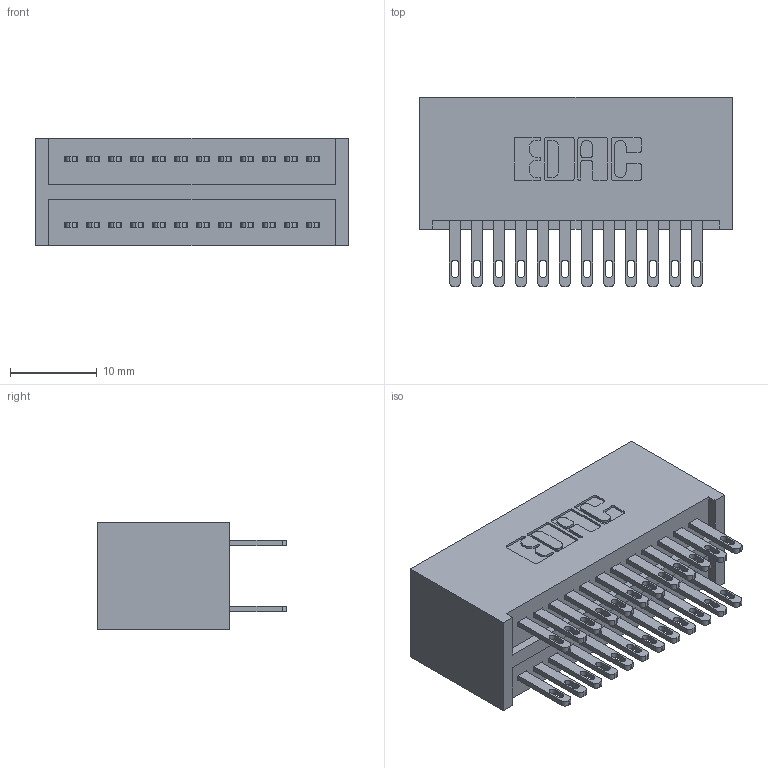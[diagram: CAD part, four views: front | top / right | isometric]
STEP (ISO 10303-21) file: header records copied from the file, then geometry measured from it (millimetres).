
FILE_DESCRIPTION (( 'STEP AP203' ), '1' );
FILE_NAME ('325-024-500-201.STEP', '2020-02-24T17:46:23', ( '' ), ( '' ), 'SwSTEP 2.0', 'SolidWorks 2016', '' );
FILE_SCHEMA (( 'CONFIG_CONTROL_DESIGN' ));
Length unit declared in the file: inch
Products named in the file (3): 325 Part_Lugless; 325-024-500-201; 325-292-001_325-293-100
Assembly tree (25 placements, depth 2):
  325-024-500-201
    325 Part_Lugless
    325-292-001_325-293-100  x24
Bounding box: 36.12 x 21.84 x 12.45 mm (x, y, z)
Volume: 5073.1 mm3; surface area: 6340.9 mm2
Topology: 25 solids, 25 shells, 1258 faces, 3815 edges, 2542 vertices
Faces by surface type: plane 786, cylinder 472
Entity records: 11253 total; most frequent: CARTESIAN_POINT 1898, ORIENTED_EDGE 1834, DIRECTION 1669, EDGE_CURVE 917, VECTOR 793, LINE 793, VERTEX_POINT 610, AXIS2_PLACEMENT_3D 438
